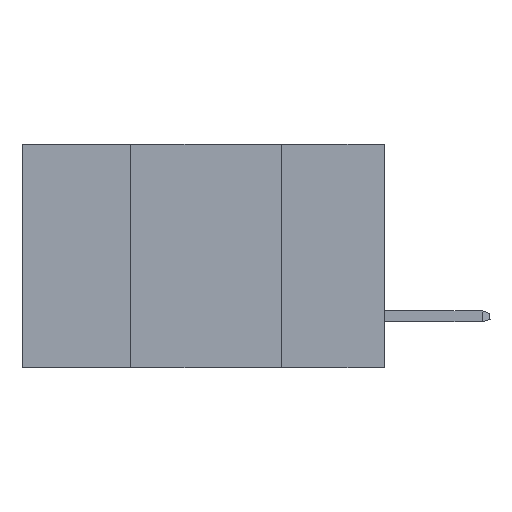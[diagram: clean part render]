
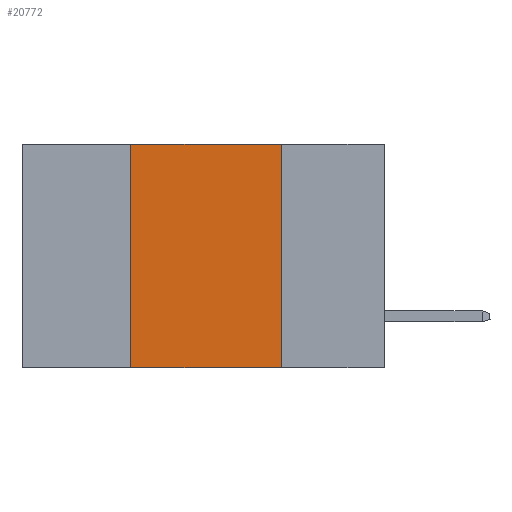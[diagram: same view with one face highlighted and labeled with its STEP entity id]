
A CAD part, left-side view. The second image highlights one B-rep face of the part: STEP entity #20772.
In plain terms, the highlighted planar face has unit normal (-1, 0, 0).
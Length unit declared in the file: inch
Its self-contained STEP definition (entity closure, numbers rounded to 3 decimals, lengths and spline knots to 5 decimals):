
#155 = DIRECTION ( 'NONE',  ( 1., 0., 0. ) ) ;
#789 = LINE ( 'NONE', #1678, #8184 ) ;
#1678 = CARTESIAN_POINT ( 'NONE',  ( 0., 0.6, -0.37 ) ) ;
#1709 = VERTEX_POINT ( 'NONE', #2977 ) ;
#1779 = CARTESIAN_POINT ( 'NONE',  ( 0., 0.6, 0. ) ) ;
#2348 = VERTEX_POINT ( 'NONE', #24452 ) ;
#2977 = CARTESIAN_POINT ( 'NONE',  ( 0., 0.17, 0. ) ) ;
#2999 = DIRECTION ( 'NONE',  ( 0., 0., -1. ) ) ;
#3048 = ORIENTED_EDGE ( 'NONE', *, *, #12367, .F. ) ;
#4825 = VECTOR ( 'NONE', #2999, 39.37008 ) ;
#4959 = VERTEX_POINT ( 'NONE', #20959 ) ;
#4975 = FACE_OUTER_BOUND ( 'NONE', #11868, .T. ) ;
#5007 = ORIENTED_EDGE ( 'NONE', *, *, #9711, .T. ) ;
#5923 = DIRECTION ( 'NONE',  ( 0., 0., -1. ) ) ;
#6759 = CARTESIAN_POINT ( 'NONE',  ( 0., 0.42, 0. ) ) ;
#7625 = DIRECTION ( 'NONE',  ( 0., -1., 0. ) ) ;
#7894 = PLANE ( 'NONE',  #16876 ) ;
#8184 = VECTOR ( 'NONE', #24989, 39.37008 ) ;
#9496 = CARTESIAN_POINT ( 'NONE',  ( 0., 0.42, 0. ) ) ;
#9711 = EDGE_CURVE ( 'NONE', #4959, #2348, #789, .T. ) ;
#11357 = EDGE_CURVE ( 'NONE', #1709, #2348, #14288, .T. ) ;
#11763 = ORIENTED_EDGE ( 'NONE', *, *, #21583, .F. ) ;
#11868 = EDGE_LOOP ( 'NONE', ( #12165, #11763, #3048, #5007 ) ) ;
#12165 = ORIENTED_EDGE ( 'NONE', *, *, #11357, .F. ) ;
#12367 = EDGE_CURVE ( 'NONE', #4959, #13919, #24556, .T. ) ;
#13919 = VERTEX_POINT ( 'NONE', #6759 ) ;
#14288 = LINE ( 'NONE', #20360, #4825 ) ;
#15638 = CARTESIAN_POINT ( 'NONE',  ( 0., 0.6, 0. ) ) ;
#16876 = AXIS2_PLACEMENT_3D ( 'NONE', #15638, #155, #5923 ) ;
#20360 = CARTESIAN_POINT ( 'NONE',  ( 0., 0.17, 0. ) ) ;
#20772 = ADVANCED_FACE ( 'NONE', ( #4975 ), #7894, .F. ) ;
#20959 = CARTESIAN_POINT ( 'NONE',  ( 0., 0.42, -0.37 ) ) ;
#21328 = DIRECTION ( 'NONE',  ( 0., 0., 1. ) ) ;
#21583 = EDGE_CURVE ( 'NONE', #13919, #1709, #21750, .T. ) ;
#21750 = LINE ( 'NONE', #1779, #23881 ) ;
#23881 = VECTOR ( 'NONE', #7625, 39.37008 ) ;
#23950 = VECTOR ( 'NONE', #21328, 39.37008 ) ;
#24452 = CARTESIAN_POINT ( 'NONE',  ( 0., 0.17, -0.37 ) ) ;
#24556 = LINE ( 'NONE', #9496, #23950 ) ;
#24989 = DIRECTION ( 'NONE',  ( 0., -1., 0. ) ) ;
